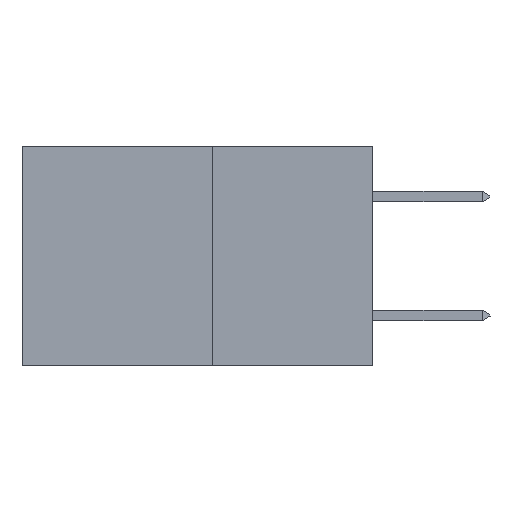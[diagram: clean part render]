
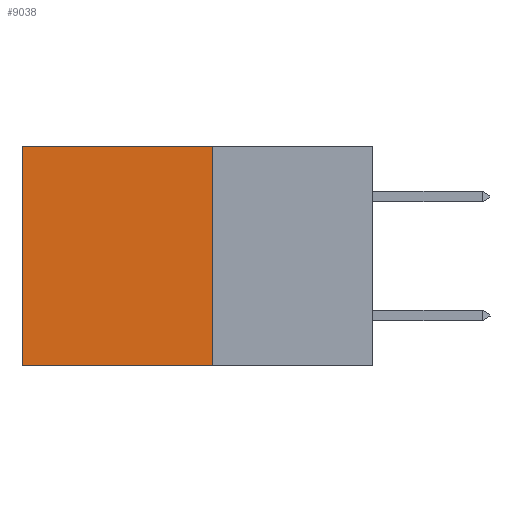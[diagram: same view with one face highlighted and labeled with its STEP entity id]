
A CAD part, left-side view. The second image highlights one B-rep face of the part: STEP entity #9038.
In plain terms, the highlighted planar face has unit normal (-1, 0, 0).
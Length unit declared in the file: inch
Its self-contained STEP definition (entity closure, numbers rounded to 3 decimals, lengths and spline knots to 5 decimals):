
#229 = VERTEX_POINT ( 'NONE', #13128 ) ;
#1324 = PLANE ( 'NONE',  #4304 ) ;
#1371 = DIRECTION ( 'NONE',  ( 0., 0., -1. ) ) ;
#1763 = CARTESIAN_POINT ( 'NONE',  ( 0.277, 0.27, -0.37 ) ) ;
#2519 = ORIENTED_EDGE ( 'NONE', *, *, #11653, .F. ) ;
#3003 = LINE ( 'NONE', #1763, #8333 ) ;
#3612 = DIRECTION ( 'NONE',  ( 0., 0., -1. ) ) ;
#4304 = AXIS2_PLACEMENT_3D ( 'NONE', #4512, #7759, #1371 ) ;
#4480 = VECTOR ( 'NONE', #12237, 39.37008 ) ;
#4512 = CARTESIAN_POINT ( 'NONE',  ( 0.277, 0.27, -0.37 ) ) ;
#4943 = ORIENTED_EDGE ( 'NONE', *, *, #12857, .F. ) ;
#5159 = LINE ( 'NONE', #13289, #4480 ) ;
#5504 = LINE ( 'NONE', #6063, #11212 ) ;
#5580 = VERTEX_POINT ( 'NONE', #10483 ) ;
#5909 = ORIENTED_EDGE ( 'NONE', *, *, #12872, .T. ) ;
#6063 = CARTESIAN_POINT ( 'NONE',  ( 0.277, 0.59, -0.37 ) ) ;
#6669 = EDGE_LOOP ( 'NONE', ( #5909, #4943, #2519, #12280 ) ) ;
#7133 = DIRECTION ( 'NONE',  ( 0., 0., -1. ) ) ;
#7759 = DIRECTION ( 'NONE',  ( 1., 0., 0. ) ) ;
#8333 = VECTOR ( 'NONE', #10300, 39.37008 ) ;
#8737 = CARTESIAN_POINT ( 'NONE',  ( 0.277, 0.59, -0.37 ) ) ;
#8850 = VECTOR ( 'NONE', #3612, 39.37008 ) ;
#8939 = CARTESIAN_POINT ( 'NONE',  ( 0.277, 0.27, -0.37 ) ) ;
#8990 = FACE_OUTER_BOUND ( 'NONE', #6669, .T. ) ;
#9038 = ADVANCED_FACE ( 'NONE', ( #8990 ), #1324, .F. ) ;
#9184 = EDGE_CURVE ( 'NONE', #12665, #5580, #5159, .T. ) ;
#10300 = DIRECTION ( 'NONE',  ( 0., 1., 0. ) ) ;
#10483 = CARTESIAN_POINT ( 'NONE',  ( 0.277, 0.59, 0. ) ) ;
#11212 = VECTOR ( 'NONE', #7133, 39.37008 ) ;
#11653 = EDGE_CURVE ( 'NONE', #12665, #229, #12093, .T. ) ;
#12093 = LINE ( 'NONE', #8939, #8850 ) ;
#12181 = VERTEX_POINT ( 'NONE', #8737 ) ;
#12237 = DIRECTION ( 'NONE',  ( 0., 1., 0. ) ) ;
#12280 = ORIENTED_EDGE ( 'NONE', *, *, #9184, .T. ) ;
#12665 = VERTEX_POINT ( 'NONE', #13268 ) ;
#12857 = EDGE_CURVE ( 'NONE', #229, #12181, #3003, .T. ) ;
#12872 = EDGE_CURVE ( 'NONE', #5580, #12181, #5504, .T. ) ;
#13128 = CARTESIAN_POINT ( 'NONE',  ( 0.277, 0.27, -0.37 ) ) ;
#13268 = CARTESIAN_POINT ( 'NONE',  ( 0.277, 0.27, 0. ) ) ;
#13289 = CARTESIAN_POINT ( 'NONE',  ( 0.277, 0.27, 0. ) ) ;
